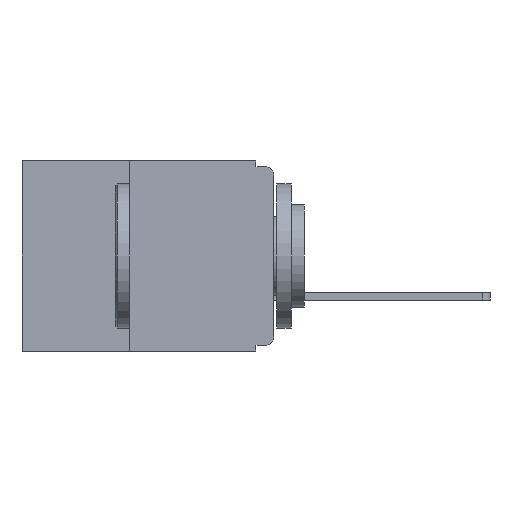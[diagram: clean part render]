
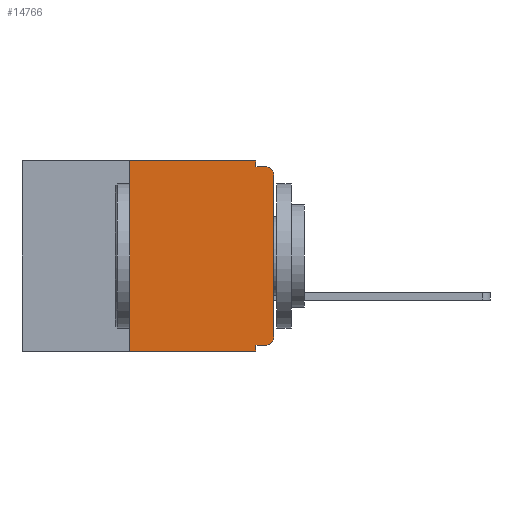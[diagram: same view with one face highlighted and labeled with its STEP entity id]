
A CAD part, left-side view. The second image highlights one B-rep face of the part: STEP entity #14766.
In plain terms, the highlighted planar face has unit normal (-1, 0, 0).
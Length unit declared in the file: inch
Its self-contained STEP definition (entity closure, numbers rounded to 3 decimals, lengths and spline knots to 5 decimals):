
#319 = CARTESIAN_POINT ( 'NONE',  ( 0., 0., -0.32 ) ) ;
#347 = DIRECTION ( 'NONE',  ( 0., 1., 0. ) ) ;
#674 = LINE ( 'NONE', #23958, #31690 ) ;
#822 = ORIENTED_EDGE ( 'NONE', *, *, #28048, .T. ) ;
#1065 = ORIENTED_EDGE ( 'NONE', *, *, #31740, .F. ) ;
#1902 = EDGE_CURVE ( 'NONE', #15648, #22218, #9788, .T. ) ;
#2049 = VECTOR ( 'NONE', #16923, 39.37008 ) ;
#2166 = EDGE_CURVE ( 'NONE', #8372, #17285, #13619, .T. ) ;
#2406 = CARTESIAN_POINT ( 'NONE',  ( 0., 0.031, -0.01 ) ) ;
#2581 = VECTOR ( 'NONE', #4848, 39.37008 ) ;
#2914 = LINE ( 'NONE', #12125, #2581 ) ;
#4848 = DIRECTION ( 'NONE',  ( 0., 0., 1. ) ) ;
#5042 = ORIENTED_EDGE ( 'NONE', *, *, #7047, .F. ) ;
#5717 = CARTESIAN_POINT ( 'NONE',  ( 0., 0.437, 0. ) ) ;
#5946 = CARTESIAN_POINT ( 'NONE',  ( 0., 0.015, -0.32 ) ) ;
#6197 = EDGE_CURVE ( 'NONE', #24973, #10906, #9114, .T. ) ;
#6665 = CARTESIAN_POINT ( 'NONE',  ( 0., 0., -0.01 ) ) ;
#7047 = EDGE_CURVE ( 'NONE', #24973, #15648, #16757, .T. ) ;
#7241 = VERTEX_POINT ( 'NONE', #27582 ) ;
#8226 = LINE ( 'NONE', #6665, #26969 ) ;
#8236 = DIRECTION ( 'NONE',  ( 1., 0., 0. ) ) ;
#8372 = VERTEX_POINT ( 'NONE', #30859 ) ;
#8524 = VERTEX_POINT ( 'NONE', #29165 ) ;
#9114 = CIRCLE ( 'NONE', #28881, 0.015 ) ;
#9335 = DIRECTION ( 'NONE',  ( 0., -1., 0. ) ) ;
#9653 = CARTESIAN_POINT ( 'NONE',  ( 0., 0.437, -0.33 ) ) ;
#9788 = LINE ( 'NONE', #25215, #26975 ) ;
#10580 = CIRCLE ( 'NONE', #10886, 0.015 ) ;
#10611 = PLANE ( 'NONE',  #12139 ) ;
#10886 = AXIS2_PLACEMENT_3D ( 'NONE', #26364, #11753, #28788 ) ;
#10906 = VERTEX_POINT ( 'NONE', #31433 ) ;
#11072 = CARTESIAN_POINT ( 'NONE',  ( 0., 0.031, 0. ) ) ;
#11384 = DIRECTION ( 'NONE',  ( 0., 0., -1. ) ) ;
#11585 = DIRECTION ( 'NONE',  ( 0., 0., -1. ) ) ;
#11595 = DIRECTION ( 'NONE',  ( -1., 0., 0. ) ) ;
#11624 = CARTESIAN_POINT ( 'NONE',  ( 0., 0.015, -0.305 ) ) ;
#11753 = DIRECTION ( 'NONE',  ( -1., 0., 0. ) ) ;
#11976 = CARTESIAN_POINT ( 'NONE',  ( 0., 0.031, -0.32 ) ) ;
#12125 = CARTESIAN_POINT ( 'NONE',  ( 0., 0., 0. ) ) ;
#12139 = AXIS2_PLACEMENT_3D ( 'NONE', #5717, #8236, #25339 ) ;
#12199 = VERTEX_POINT ( 'NONE', #29585 ) ;
#12596 = LINE ( 'NONE', #27092, #24789 ) ;
#12636 = ORIENTED_EDGE ( 'NONE', *, *, #1902, .F. ) ;
#13110 = ORIENTED_EDGE ( 'NONE', *, *, #2166, .F. ) ;
#13151 = ORIENTED_EDGE ( 'NONE', *, *, #6197, .T. ) ;
#13619 = LINE ( 'NONE', #11072, #31458 ) ;
#13883 = ORIENTED_EDGE ( 'NONE', *, *, #26934, .F. ) ;
#14061 = FACE_OUTER_BOUND ( 'NONE', #25282, .T. ) ;
#14517 = EDGE_CURVE ( 'NONE', #12199, #22218, #21223, .T. ) ;
#14766 = ADVANCED_FACE ( 'NONE', ( #14061 ), #10611, .F. ) ;
#14910 = DIRECTION ( 'NONE',  ( 0., 0., 1. ) ) ;
#15648 = VERTEX_POINT ( 'NONE', #11976 ) ;
#16316 = ORIENTED_EDGE ( 'NONE', *, *, #28796, .T. ) ;
#16757 = LINE ( 'NONE', #319, #29697 ) ;
#16923 = DIRECTION ( 'NONE',  ( 0., -1., 0. ) ) ;
#17285 = VERTEX_POINT ( 'NONE', #2406 ) ;
#19193 = CARTESIAN_POINT ( 'NONE',  ( 0., 0.015, -0.01 ) ) ;
#20272 = ORIENTED_EDGE ( 'NONE', *, *, #25442, .F. ) ;
#21223 = LINE ( 'NONE', #9653, #2049 ) ;
#21381 = VERTEX_POINT ( 'NONE', #19193 ) ;
#22218 = VERTEX_POINT ( 'NONE', #22367 ) ;
#22367 = CARTESIAN_POINT ( 'NONE',  ( 0., 0.031, -0.33 ) ) ;
#23958 = CARTESIAN_POINT ( 'NONE',  ( 0., 0.437, 0. ) ) ;
#24789 = VECTOR ( 'NONE', #14910, 39.37008 ) ;
#24973 = VERTEX_POINT ( 'NONE', #5946 ) ;
#25215 = CARTESIAN_POINT ( 'NONE',  ( 0., 0.031, -0.33 ) ) ;
#25282 = EDGE_LOOP ( 'NONE', ( #16316, #822, #1065, #13110, #20272, #13883, #28249, #12636, #5042, #13151 ) ) ;
#25339 = DIRECTION ( 'NONE',  ( 0., 0., -1. ) ) ;
#25442 = EDGE_CURVE ( 'NONE', #7241, #8372, #674, .T. ) ;
#26364 = CARTESIAN_POINT ( 'NONE',  ( 0., 0.015, -0.025 ) ) ;
#26934 = EDGE_CURVE ( 'NONE', #12199, #7241, #12596, .T. ) ;
#26969 = VECTOR ( 'NONE', #31105, 39.37008 ) ;
#26975 = VECTOR ( 'NONE', #29225, 39.37008 ) ;
#27092 = CARTESIAN_POINT ( 'NONE',  ( 0., 0.25, -0.33 ) ) ;
#27582 = CARTESIAN_POINT ( 'NONE',  ( 0., 0.25, 0. ) ) ;
#28048 = EDGE_CURVE ( 'NONE', #8524, #21381, #10580, .T. ) ;
#28249 = ORIENTED_EDGE ( 'NONE', *, *, #14517, .T. ) ;
#28788 = DIRECTION ( 'NONE',  ( 0., 0., -1. ) ) ;
#28796 = EDGE_CURVE ( 'NONE', #10906, #8524, #2914, .T. ) ;
#28881 = AXIS2_PLACEMENT_3D ( 'NONE', #11624, #11595, #11585 ) ;
#29165 = CARTESIAN_POINT ( 'NONE',  ( 0., 0., -0.025 ) ) ;
#29225 = DIRECTION ( 'NONE',  ( 0., 0., -1. ) ) ;
#29585 = CARTESIAN_POINT ( 'NONE',  ( 0., 0.25, -0.33 ) ) ;
#29697 = VECTOR ( 'NONE', #347, 39.37008 ) ;
#30859 = CARTESIAN_POINT ( 'NONE',  ( 0., 0.031, 0. ) ) ;
#31105 = DIRECTION ( 'NONE',  ( 0., -1., 0. ) ) ;
#31433 = CARTESIAN_POINT ( 'NONE',  ( 0., 0., -0.305 ) ) ;
#31458 = VECTOR ( 'NONE', #11384, 39.37008 ) ;
#31690 = VECTOR ( 'NONE', #9335, 39.37008 ) ;
#31740 = EDGE_CURVE ( 'NONE', #17285, #21381, #8226, .T. ) ;
